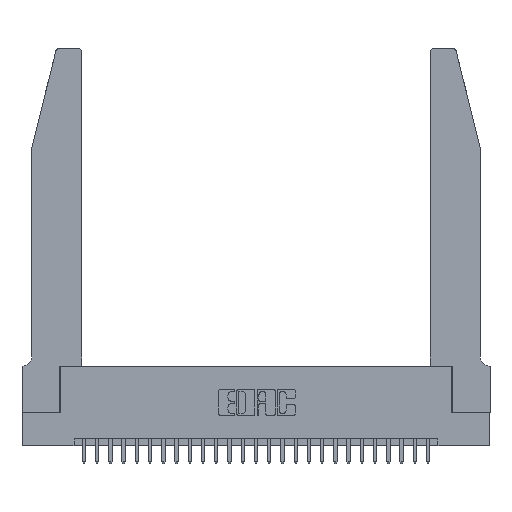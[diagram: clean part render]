
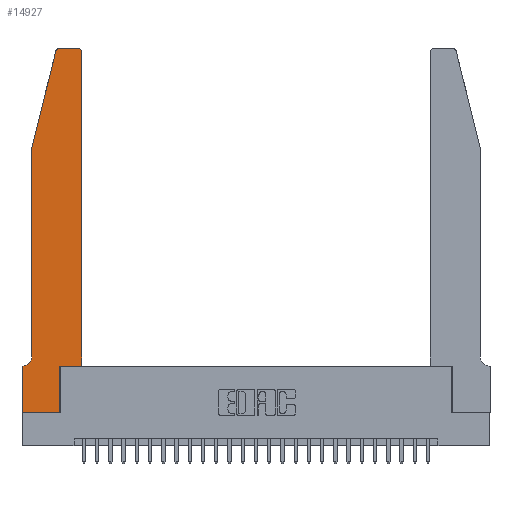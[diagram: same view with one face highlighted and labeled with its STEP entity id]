
A CAD part, top view. The second image highlights one B-rep face of the part: STEP entity #14927.
In plain terms, the highlighted planar face has unit normal (0, 0, 1).
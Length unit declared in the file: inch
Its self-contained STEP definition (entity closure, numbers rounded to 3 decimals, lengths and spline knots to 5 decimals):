
#150 = ORIENTED_EDGE ( 'NONE', *, *, #6785, .T. ) ;
#238 = LINE ( 'NONE', #21652, #4761 ) ;
#714 = LINE ( 'NONE', #20639, #23033 ) ;
#739 = CIRCLE ( 'NONE', #6218, 0.07 ) ;
#1069 = EDGE_CURVE ( 'NONE', #11020, #27636, #4944, .T. ) ;
#1074 = LINE ( 'NONE', #9188, #23379 ) ;
#1588 = AXIS2_PLACEMENT_3D ( 'NONE', #22983, #25170, #12401 ) ;
#2157 = LINE ( 'NONE', #24869, #7360 ) ;
#2548 = EDGE_CURVE ( 'NONE', #27636, #6102, #739, .T. ) ;
#3008 = CARTESIAN_POINT ( 'NONE',  ( 0., 0., 0.37 ) ) ;
#4359 = CARTESIAN_POINT ( 'NONE',  ( 0.2605, 2.75, 0.37 ) ) ;
#4463 = EDGE_CURVE ( 'NONE', #18063, #7094, #19957, .T. ) ;
#4761 = VECTOR ( 'NONE', #17462, 39.37008 ) ;
#4944 = LINE ( 'NONE', #13362, #10776 ) ;
#5190 = CARTESIAN_POINT ( 'NONE',  ( 0.25487, 2.72718, 0.37 ) ) ;
#5883 = DIRECTION ( 'NONE',  ( 0., -1., 0. ) ) ;
#6102 = VERTEX_POINT ( 'NONE', #19724 ) ;
#6135 = LINE ( 'NONE', #25507, #11915 ) ;
#6218 = AXIS2_PLACEMENT_3D ( 'NONE', #23524, #10770, #25714 ) ;
#6775 = CIRCLE ( 'NONE', #12005, 0.03 ) ;
#6785 = EDGE_CURVE ( 'NONE', #16448, #19177, #1074, .T. ) ;
#6918 = EDGE_CURVE ( 'NONE', #19177, #27142, #16389, .T. ) ;
#7019 = EDGE_CURVE ( 'NONE', #13620, #11020, #714, .T. ) ;
#7094 = VERTEX_POINT ( 'NONE', #12381 ) ;
#7360 = VECTOR ( 'NONE', #27026, 39.37008 ) ;
#7572 = CARTESIAN_POINT ( 'NONE',  ( 0.284, 2.72, 0.37 ) ) ;
#8050 = VERTEX_POINT ( 'NONE', #27891 ) ;
#8065 = PLANE ( 'NONE',  #1588 ) ;
#8441 = CARTESIAN_POINT ( 'NONE',  ( 0.0755, 2., 0.37 ) ) ;
#9186 = EDGE_CURVE ( 'NONE', #6102, #16448, #238, .T. ) ;
#9188 = CARTESIAN_POINT ( 'NONE',  ( 0., 0., 0.37 ) ) ;
#9214 = ORIENTED_EDGE ( 'NONE', *, *, #13143, .T. ) ;
#9749 = DIRECTION ( 'NONE',  ( 1., 0., 0. ) ) ;
#9765 = CARTESIAN_POINT ( 'NONE',  ( 0.4505, 2.72, 0.37 ) ) ;
#10549 = CIRCLE ( 'NONE', #11246, 0.03 ) ;
#10574 = ORIENTED_EDGE ( 'NONE', *, *, #22686, .T. ) ;
#10770 = DIRECTION ( 'NONE',  ( 0., 0., -1. ) ) ;
#10776 = VECTOR ( 'NONE', #5883, 39.37008 ) ;
#11020 = VERTEX_POINT ( 'NONE', #8441 ) ;
#11246 = AXIS2_PLACEMENT_3D ( 'NONE', #12718, #27629, #14833 ) ;
#11309 = EDGE_CURVE ( 'NONE', #7094, #13620, #6775, .T. ) ;
#11439 = CARTESIAN_POINT ( 'NONE',  ( 0., 0., 0.37 ) ) ;
#11522 = ORIENTED_EDGE ( 'NONE', *, *, #9186, .T. ) ;
#11542 = EDGE_LOOP ( 'NONE', ( #23537, #22335, #25446, #13254, #16715, #11522, #150, #24875, #13006, #13581, #9214, #10574 ) ) ;
#11819 = DIRECTION ( 'NONE',  ( 1., 0., 0. ) ) ;
#11915 = VECTOR ( 'NONE', #12733, 39.37008 ) ;
#12005 = AXIS2_PLACEMENT_3D ( 'NONE', #7572, #22505, #9749 ) ;
#12339 = VECTOR ( 'NONE', #25898, 39.37008 ) ;
#12381 = CARTESIAN_POINT ( 'NONE',  ( 0.284, 2.75, 0.37 ) ) ;
#12401 = DIRECTION ( 'NONE',  ( 1., 0., 0. ) ) ;
#12718 = CARTESIAN_POINT ( 'NONE',  ( 0.4205, 2.72, 0.37 ) ) ;
#12733 = DIRECTION ( 'NONE',  ( 0., 1., 0. ) ) ;
#12917 = CARTESIAN_POINT ( 'NONE',  ( 0.0755, 0.42, 0.37 ) ) ;
#13006 = ORIENTED_EDGE ( 'NONE', *, *, #15679, .T. ) ;
#13033 = CARTESIAN_POINT ( 'NONE',  ( 0.2865, 0., 0.37 ) ) ;
#13143 = EDGE_CURVE ( 'NONE', #24915, #26782, #2157, .T. ) ;
#13254 = ORIENTED_EDGE ( 'NONE', *, *, #1069, .T. ) ;
#13362 = CARTESIAN_POINT ( 'NONE',  ( 0.0755, 2., 0.37 ) ) ;
#13581 = ORIENTED_EDGE ( 'NONE', *, *, #21085, .T. ) ;
#13620 = VERTEX_POINT ( 'NONE', #5190 ) ;
#14833 = DIRECTION ( 'NONE',  ( 1., 0., 0. ) ) ;
#14927 = ADVANCED_FACE ( 'NONE', ( #27928 ), #8065, .T. ) ;
#15611 = DIRECTION ( 'NONE',  ( 0., -1., 0. ) ) ;
#15679 = EDGE_CURVE ( 'NONE', #27142, #8050, #6135, .T. ) ;
#16360 = DIRECTION ( 'NONE',  ( -0.239, -0.971, 0. ) ) ;
#16389 = LINE ( 'NONE', #3008, #21357 ) ;
#16448 = VERTEX_POINT ( 'NONE', #21685 ) ;
#16715 = ORIENTED_EDGE ( 'NONE', *, *, #2548, .T. ) ;
#17462 = DIRECTION ( 'NONE',  ( -1., 0., 0. ) ) ;
#18063 = VERTEX_POINT ( 'NONE', #22210 ) ;
#19177 = VERTEX_POINT ( 'NONE', #11439 ) ;
#19724 = CARTESIAN_POINT ( 'NONE',  ( 0.0055, 0.35, 0.37 ) ) ;
#19957 = LINE ( 'NONE', #4359, #12339 ) ;
#20631 = CARTESIAN_POINT ( 'NONE',  ( 0.4505, 0.35, 0.37 ) ) ;
#20639 = CARTESIAN_POINT ( 'NONE',  ( 0.0755, 2., 0.37 ) ) ;
#20934 = VECTOR ( 'NONE', #27108, 39.37008 ) ;
#21085 = EDGE_CURVE ( 'NONE', #8050, #24915, #26644, .T. ) ;
#21357 = VECTOR ( 'NONE', #11819, 39.37008 ) ;
#21652 = CARTESIAN_POINT ( 'NONE',  ( 0.0755, 0.35, 0.37 ) ) ;
#21685 = CARTESIAN_POINT ( 'NONE',  ( 0., 0.35, 0.37 ) ) ;
#22210 = CARTESIAN_POINT ( 'NONE',  ( 0.4205, 2.75, 0.37 ) ) ;
#22335 = ORIENTED_EDGE ( 'NONE', *, *, #11309, .T. ) ;
#22505 = DIRECTION ( 'NONE',  ( 0., 0., 1. ) ) ;
#22686 = EDGE_CURVE ( 'NONE', #26782, #18063, #10549, .T. ) ;
#22983 = CARTESIAN_POINT ( 'NONE',  ( 0., 0.35, 0.37 ) ) ;
#23033 = VECTOR ( 'NONE', #16360, 39.37008 ) ;
#23379 = VECTOR ( 'NONE', #15611, 39.37008 ) ;
#23524 = CARTESIAN_POINT ( 'NONE',  ( 0.0055, 0.42, 0.37 ) ) ;
#23537 = ORIENTED_EDGE ( 'NONE', *, *, #4463, .T. ) ;
#24869 = CARTESIAN_POINT ( 'NONE',  ( 0.4505, 0.35, 0.37 ) ) ;
#24875 = ORIENTED_EDGE ( 'NONE', *, *, #6918, .T. ) ;
#24899 = CARTESIAN_POINT ( 'NONE',  ( 0.4505, 0.35, 0.37 ) ) ;
#24915 = VERTEX_POINT ( 'NONE', #24899 ) ;
#25170 = DIRECTION ( 'NONE',  ( 0., 0., 1. ) ) ;
#25446 = ORIENTED_EDGE ( 'NONE', *, *, #7019, .T. ) ;
#25507 = CARTESIAN_POINT ( 'NONE',  ( 0.2865, 0.35, 0.37 ) ) ;
#25714 = DIRECTION ( 'NONE',  ( -1., 0., 0. ) ) ;
#25898 = DIRECTION ( 'NONE',  ( -1., 0., 0. ) ) ;
#26644 = LINE ( 'NONE', #20631, #20934 ) ;
#26782 = VERTEX_POINT ( 'NONE', #9765 ) ;
#27026 = DIRECTION ( 'NONE',  ( 0., 1., 0. ) ) ;
#27108 = DIRECTION ( 'NONE',  ( 1., 0., 0. ) ) ;
#27142 = VERTEX_POINT ( 'NONE', #13033 ) ;
#27629 = DIRECTION ( 'NONE',  ( 0., 0., 1. ) ) ;
#27636 = VERTEX_POINT ( 'NONE', #12917 ) ;
#27891 = CARTESIAN_POINT ( 'NONE',  ( 0.2865, 0.35, 0.37 ) ) ;
#27928 = FACE_OUTER_BOUND ( 'NONE', #11542, .T. ) ;
